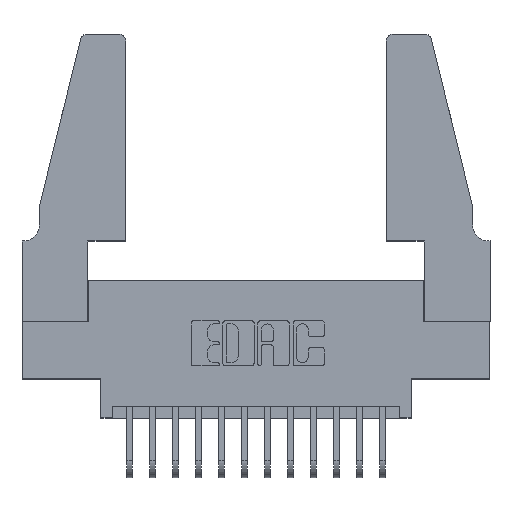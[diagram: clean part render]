
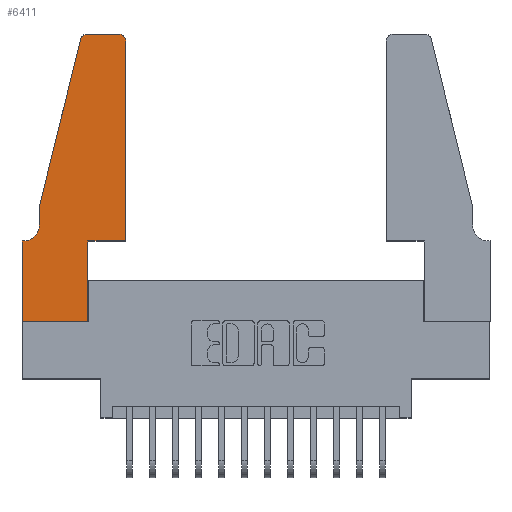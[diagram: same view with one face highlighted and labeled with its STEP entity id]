
A CAD part, top view. The second image highlights one B-rep face of the part: STEP entity #6411.
In plain terms, the highlighted planar face has unit normal (0, 0, 1).
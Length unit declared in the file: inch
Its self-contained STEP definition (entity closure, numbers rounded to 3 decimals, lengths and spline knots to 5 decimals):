
#33 = DIRECTION ( 'NONE',  ( 0., -1., 0. ) ) ;
#38 = LINE ( 'NONE', #9656, #13116 ) ;
#105 = ORIENTED_EDGE ( 'NONE', *, *, #1884, .T. ) ;
#278 = LINE ( 'NONE', #4035, #15424 ) ;
#381 = EDGE_CURVE ( 'NONE', #6028, #9352, #3199, .T. ) ;
#384 = PLANE ( 'NONE',  #8225 ) ;
#536 = EDGE_LOOP ( 'NONE', ( #3149, #5748, #6583, #2070, #3535, #6067, #105, #2247, #10430, #4425, #5680, #14008 ) ) ;
#560 = LINE ( 'NONE', #14521, #3738 ) ;
#646 = LINE ( 'NONE', #4900, #12995 ) ;
#696 = EDGE_CURVE ( 'NONE', #9352, #3837, #13860, .T. ) ;
#1020 = CARTESIAN_POINT ( 'NONE',  ( 0.2605, 1.25, 0.37 ) ) ;
#1075 = CARTESIAN_POINT ( 'NONE',  ( 0.4505, 0.35, 0.37 ) ) ;
#1501 = VECTOR ( 'NONE', #10654, 39.37008 ) ;
#1532 = CARTESIAN_POINT ( 'NONE',  ( 0., 0.35, 0.37 ) ) ;
#1558 = VERTEX_POINT ( 'NONE', #11348 ) ;
#1884 = EDGE_CURVE ( 'NONE', #11520, #6028, #3345, .T. ) ;
#2070 = ORIENTED_EDGE ( 'NONE', *, *, #4511, .T. ) ;
#2082 = CARTESIAN_POINT ( 'NONE',  ( 0.25487, 1.22718, 0.37 ) ) ;
#2218 = EDGE_CURVE ( 'NONE', #4238, #4574, #4815, .T. ) ;
#2247 = ORIENTED_EDGE ( 'NONE', *, *, #381, .T. ) ;
#2467 = EDGE_CURVE ( 'NONE', #3183, #3500, #10465, .T. ) ;
#2744 = DIRECTION ( 'NONE',  ( 1., 0., 0. ) ) ;
#3051 = EDGE_CURVE ( 'NONE', #4574, #3183, #8960, .T. ) ;
#3052 = CARTESIAN_POINT ( 'NONE',  ( 0.0755, 0.42, 0.37 ) ) ;
#3068 = CARTESIAN_POINT ( 'NONE',  ( 0.4205, 1.22, 0.37 ) ) ;
#3149 = ORIENTED_EDGE ( 'NONE', *, *, #3051, .T. ) ;
#3183 = VERTEX_POINT ( 'NONE', #12031 ) ;
#3199 = LINE ( 'NONE', #11664, #6005 ) ;
#3345 = LINE ( 'NONE', #8385, #9715 ) ;
#3500 = VERTEX_POINT ( 'NONE', #2082 ) ;
#3535 = ORIENTED_EDGE ( 'NONE', *, *, #10427, .T. ) ;
#3540 = CARTESIAN_POINT ( 'NONE',  ( 0.2865, 0.35, 0.37 ) ) ;
#3650 = DIRECTION ( 'NONE',  ( 0., 0., 1. ) ) ;
#3738 = VECTOR ( 'NONE', #7379, 39.37008 ) ;
#3837 = VERTEX_POINT ( 'NONE', #14504 ) ;
#4035 = CARTESIAN_POINT ( 'NONE',  ( 0.0755, 0.5, 0.37 ) ) ;
#4238 = VERTEX_POINT ( 'NONE', #10486 ) ;
#4288 = DIRECTION ( 'NONE',  ( 1., 0., 0. ) ) ;
#4425 = ORIENTED_EDGE ( 'NONE', *, *, #9676, .T. ) ;
#4511 = EDGE_CURVE ( 'NONE', #1558, #15092, #278, .T. ) ;
#4574 = VERTEX_POINT ( 'NONE', #8972 ) ;
#4815 = CIRCLE ( 'NONE', #11512, 0.03 ) ;
#4899 = EDGE_CURVE ( 'NONE', #9015, #11520, #646, .T. ) ;
#4900 = CARTESIAN_POINT ( 'NONE',  ( 0.0755, 0.35, 0.37 ) ) ;
#5680 = ORIENTED_EDGE ( 'NONE', *, *, #9803, .T. ) ;
#5748 = ORIENTED_EDGE ( 'NONE', *, *, #2467, .T. ) ;
#5758 = VECTOR ( 'NONE', #8255, 39.37008 ) ;
#5813 = LINE ( 'NONE', #1075, #1501 ) ;
#6005 = VECTOR ( 'NONE', #6809, 39.37008 ) ;
#6028 = VERTEX_POINT ( 'NONE', #9406 ) ;
#6067 = ORIENTED_EDGE ( 'NONE', *, *, #4899, .T. ) ;
#6116 = DIRECTION ( 'NONE',  ( 0., 0., -1. ) ) ;
#6120 = DIRECTION ( 'NONE',  ( -1., 0., 0. ) ) ;
#6411 = ADVANCED_FACE ( 'NONE', ( #13877 ), #384, .T. ) ;
#6439 = DIRECTION ( 'NONE',  ( 0., -1., 0. ) ) ;
#6583 = ORIENTED_EDGE ( 'NONE', *, *, #10467, .T. ) ;
#6809 = DIRECTION ( 'NONE',  ( 1., 0., 0. ) ) ;
#7379 = DIRECTION ( 'NONE',  ( -0.239, -0.971, 0. ) ) ;
#8225 = AXIS2_PLACEMENT_3D ( 'NONE', #8751, #9955, #2744 ) ;
#8255 = DIRECTION ( 'NONE',  ( -1., 0., 0. ) ) ;
#8385 = CARTESIAN_POINT ( 'NONE',  ( 0., 0., 0.37 ) ) ;
#8674 = VERTEX_POINT ( 'NONE', #11213 ) ;
#8751 = CARTESIAN_POINT ( 'NONE',  ( 0., 0.35, 0.37 ) ) ;
#8960 = LINE ( 'NONE', #1020, #5758 ) ;
#8972 = CARTESIAN_POINT ( 'NONE',  ( 0.4205, 1.25, 0.37 ) ) ;
#9015 = VERTEX_POINT ( 'NONE', #10761 ) ;
#9166 = AXIS2_PLACEMENT_3D ( 'NONE', #13277, #6116, #14471 ) ;
#9352 = VERTEX_POINT ( 'NONE', #10174 ) ;
#9406 = CARTESIAN_POINT ( 'NONE',  ( 0., 0., 0.37 ) ) ;
#9656 = CARTESIAN_POINT ( 'NONE',  ( 0.4505, 0.35, 0.37 ) ) ;
#9676 = EDGE_CURVE ( 'NONE', #3837, #8674, #5813, .T. ) ;
#9715 = VECTOR ( 'NONE', #33, 39.37008 ) ;
#9803 = EDGE_CURVE ( 'NONE', #8674, #4238, #38, .T. ) ;
#9955 = DIRECTION ( 'NONE',  ( 0., 0., 1. ) ) ;
#10174 = CARTESIAN_POINT ( 'NONE',  ( 0.2865, 0., 0.37 ) ) ;
#10313 = VECTOR ( 'NONE', #14305, 39.37008 ) ;
#10427 = EDGE_CURVE ( 'NONE', #15092, #9015, #10849, .T. ) ;
#10430 = ORIENTED_EDGE ( 'NONE', *, *, #696, .T. ) ;
#10465 = CIRCLE ( 'NONE', #13619, 0.03 ) ;
#10467 = EDGE_CURVE ( 'NONE', #3500, #1558, #560, .T. ) ;
#10486 = CARTESIAN_POINT ( 'NONE',  ( 0.4505, 1.22, 0.37 ) ) ;
#10654 = DIRECTION ( 'NONE',  ( 1., 0., 0. ) ) ;
#10761 = CARTESIAN_POINT ( 'NONE',  ( 0.0055, 0.35, 0.37 ) ) ;
#10814 = CARTESIAN_POINT ( 'NONE',  ( 0.284, 1.22, 0.37 ) ) ;
#10848 = DIRECTION ( 'NONE',  ( 0., 1., 0. ) ) ;
#10849 = CIRCLE ( 'NONE', #9166, 0.07 ) ;
#11213 = CARTESIAN_POINT ( 'NONE',  ( 0.4505, 0.35, 0.37 ) ) ;
#11348 = CARTESIAN_POINT ( 'NONE',  ( 0.0755, 0.5, 0.37 ) ) ;
#11435 = DIRECTION ( 'NONE',  ( 0., 0., 1. ) ) ;
#11512 = AXIS2_PLACEMENT_3D ( 'NONE', #3068, #11435, #4288 ) ;
#11520 = VERTEX_POINT ( 'NONE', #1532 ) ;
#11664 = CARTESIAN_POINT ( 'NONE',  ( 0., 0., 0.37 ) ) ;
#12005 = DIRECTION ( 'NONE',  ( 1., 0., 0. ) ) ;
#12031 = CARTESIAN_POINT ( 'NONE',  ( 0.284, 1.25, 0.37 ) ) ;
#12995 = VECTOR ( 'NONE', #6120, 39.37008 ) ;
#13116 = VECTOR ( 'NONE', #10848, 39.37008 ) ;
#13277 = CARTESIAN_POINT ( 'NONE',  ( 0.0055, 0.42, 0.37 ) ) ;
#13619 = AXIS2_PLACEMENT_3D ( 'NONE', #10814, #3650, #12005 ) ;
#13860 = LINE ( 'NONE', #3540, #10313 ) ;
#13877 = FACE_OUTER_BOUND ( 'NONE', #536, .T. ) ;
#14008 = ORIENTED_EDGE ( 'NONE', *, *, #2218, .T. ) ;
#14305 = DIRECTION ( 'NONE',  ( 0., 1., 0. ) ) ;
#14471 = DIRECTION ( 'NONE',  ( -1., 0., 0. ) ) ;
#14504 = CARTESIAN_POINT ( 'NONE',  ( 0.2865, 0.35, 0.37 ) ) ;
#14521 = CARTESIAN_POINT ( 'NONE',  ( 0.0755, 0.5, 0.37 ) ) ;
#15092 = VERTEX_POINT ( 'NONE', #3052 ) ;
#15424 = VECTOR ( 'NONE', #6439, 39.37008 ) ;
